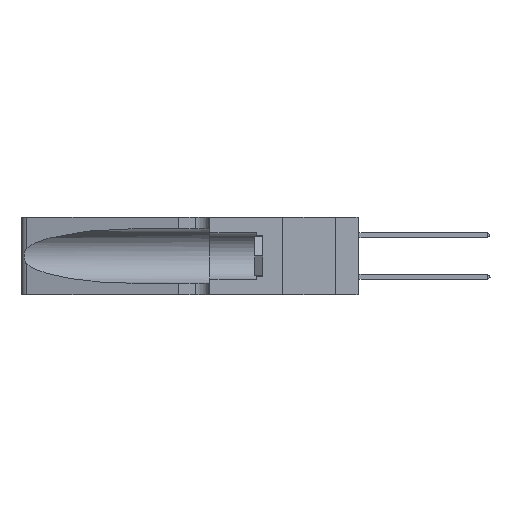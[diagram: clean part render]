
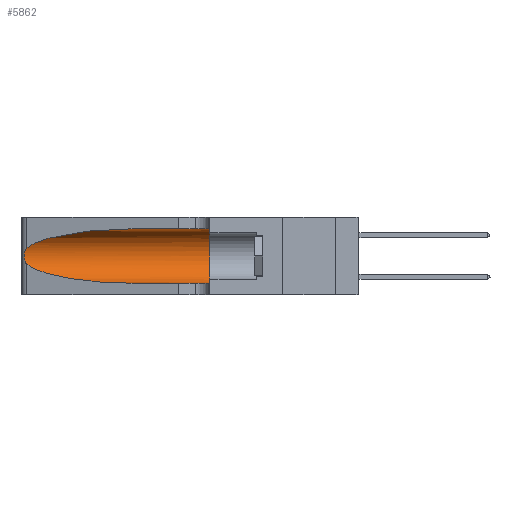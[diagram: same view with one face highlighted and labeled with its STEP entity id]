
A CAD part, left-side view. The second image highlights one B-rep face of the part: STEP entity #5862.
In plain terms, the highlighted cylindrical face has radius 3.308 mm (diameter 6.617 mm), a partial arc.
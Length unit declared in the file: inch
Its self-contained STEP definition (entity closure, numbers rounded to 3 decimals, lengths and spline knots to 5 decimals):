
#509 = CARTESIAN_POINT ( 'NONE',  ( 0.18966, 0.96281, 0.31525 ) ) ;
#884 = VECTOR ( 'NONE', #22544, 39.37008 ) ;
#1430 = ORIENTED_EDGE ( 'NONE', *, *, #12419, .T. ) ;
#1910 = LINE ( 'NONE', #32463, #884 ) ;
#2822 = AXIS2_PLACEMENT_3D ( 'NONE', #3629, #26888, #6989 ) ;
#3454 = CARTESIAN_POINT ( 'NONE',  ( 0.2373, 1.15595, 0.08982 ) ) ;
#3629 = CARTESIAN_POINT ( 'NONE',  ( 0.1305, 0.35, 0.185 ) ) ;
#3849 = CARTESIAN_POINT ( 'NONE',  ( 0.25487, 1.22718, 0.22369 ) ) ;
#4220 = CARTESIAN_POINT ( 'NONE',  ( 0.25787, 1.23484, 0.2124 ) ) ;
#4784 = ORIENTED_EDGE ( 'NONE', *, *, #43040, .T. ) ;
#4996 = EDGE_CURVE ( 'NONE', #33672, #31759, #29133, .T. ) ;
#5638 = B_SPLINE_CURVE_WITH_KNOTS ( 'NONE', 3,
 ( #17421, #37397, #24104, #4220, #27469, #7570, #30800, #10897, #34150, #14226, #37538, #17568, #40885, #20920 ),
 .UNSPECIFIED., .F., .F.,
 ( 4, 2, 2, 2, 2, 2, 4 ),
 ( 0., 0.00027, 0.00053, 0.00107, 0.0016, 0.00187, 0.00214 ),
 .UNSPECIFIED. ) ;
#5862 = ADVANCED_FACE ( 'NONE', ( #12404 ), #29058, .F. ) ;
#6635 = ORIENTED_EDGE ( 'NONE', *, *, #7661, .T. ) ;
#6989 = DIRECTION ( 'NONE',  ( 0., 0., 1. ) ) ;
#7570 = CARTESIAN_POINT ( 'NONE',  ( 0.26018, 1.23835, 0.19895 ) ) ;
#7661 = EDGE_CURVE ( 'NONE', #34881, #16072, #12007, .T. ) ;
#9265 = CARTESIAN_POINT ( 'NONE',  ( 0.1305, 1.61858, 0.31525 ) ) ;
#10110 = CARTESIAN_POINT ( 'NONE',  ( 0.25487, 1.22718, 0.14631 ) ) ;
#10220 = DIRECTION ( 'NONE',  ( 0., 0., -1. ) ) ;
#10897 = CARTESIAN_POINT ( 'NONE',  ( 0.26075, 1.23896, 0.178 ) ) ;
#11985 = EDGE_CURVE ( 'NONE', #33672, #36400, #32015, .T. ) ;
#12007 =( BOUNDED_CURVE ( )  B_SPLINE_CURVE ( 3, ( #10110, #3454, #30020, #13440 ),
 .UNSPECIFIED., .F., .F. ) 
 B_SPLINE_CURVE_WITH_KNOTS ( ( 4, 4 ),
 ( 3.44316, 4.71239 ),
 .UNSPECIFIED. ) 
 CURVE ( )  GEOMETRIC_REPRESENTATION_ITEM ( )  RATIONAL_B_SPLINE_CURVE ( ( 1., 0.87, 0.87, 1. ) ) 
 REPRESENTATION_ITEM ( '' )  );
#12404 = FACE_OUTER_BOUND ( 'NONE', #38258, .T. ) ;
#12419 = EDGE_CURVE ( 'NONE', #16072, #28475, #1910, .T. ) ;
#12459 = ORIENTED_EDGE ( 'NONE', *, *, #11985, .T. ) ;
#12831 = CARTESIAN_POINT ( 'NONE',  ( 0.1305, 0.35, 0.31525 ) ) ;
#13440 = CARTESIAN_POINT ( 'NONE',  ( 0.1305, 0.72297, 0.05475 ) ) ;
#14226 = CARTESIAN_POINT ( 'NONE',  ( 0.25856, 1.23593, 0.16098 ) ) ;
#14523 = CIRCLE ( 'NONE', #2822, 0.13025 ) ;
#16072 = VERTEX_POINT ( 'NONE', #16945 ) ;
#16945 = CARTESIAN_POINT ( 'NONE',  ( 0.1305, 0.72297, 0.05475 ) ) ;
#17421 = CARTESIAN_POINT ( 'NONE',  ( 0.25487, 1.22718, 0.22369 ) ) ;
#17568 = CARTESIAN_POINT ( 'NONE',  ( 0.25639, 1.23186, 0.15144 ) ) ;
#20098 = CARTESIAN_POINT ( 'NONE',  ( 0.1305, 1.61858, 0.185 ) ) ;
#20405 = CARTESIAN_POINT ( 'NONE',  ( 0.2373, 1.15595, 0.28018 ) ) ;
#20920 = CARTESIAN_POINT ( 'NONE',  ( 0.25487, 1.22718, 0.14631 ) ) ;
#22544 = DIRECTION ( 'NONE',  ( 0., -1., 0. ) ) ;
#24104 = CARTESIAN_POINT ( 'NONE',  ( 0.25639, 1.23184, 0.21858 ) ) ;
#26888 = DIRECTION ( 'NONE',  ( 0., 1., 0. ) ) ;
#27469 = CARTESIAN_POINT ( 'NONE',  ( 0.25854, 1.2359, 0.20912 ) ) ;
#28377 = CARTESIAN_POINT ( 'NONE',  ( 0.1305, 0.35, 0.05475 ) ) ;
#28475 = VERTEX_POINT ( 'NONE', #28377 ) ;
#29058 = CYLINDRICAL_SURFACE ( 'NONE', #32369, 0.13025 ) ;
#29133 = LINE ( 'NONE', #9265, #36973 ) ;
#30020 = CARTESIAN_POINT ( 'NONE',  ( 0.18966, 0.96281, 0.05475 ) ) ;
#30125 = DIRECTION ( 'NONE',  ( 0., -1., 0. ) ) ;
#30777 = ORIENTED_EDGE ( 'NONE', *, *, #4996, .F. ) ;
#30800 = CARTESIAN_POINT ( 'NONE',  ( 0.26075, 1.23896, 0.19203 ) ) ;
#31759 = VERTEX_POINT ( 'NONE', #12831 ) ;
#32015 =( BOUNDED_CURVE ( )  B_SPLINE_CURVE ( 3, ( #40357, #509, #20405, #3849 ),
 .UNSPECIFIED., .F., .F. ) 
 B_SPLINE_CURVE_WITH_KNOTS ( ( 4, 4 ),
 ( 1.5708, 2.84003 ),
 .UNSPECIFIED. ) 
 CURVE ( )  GEOMETRIC_REPRESENTATION_ITEM ( )  RATIONAL_B_SPLINE_CURVE ( ( 1., 0.87, 0.87, 1. ) ) 
 REPRESENTATION_ITEM ( '' )  );
#32369 = AXIS2_PLACEMENT_3D ( 'NONE', #20098, #30125, #10220 ) ;
#32463 = CARTESIAN_POINT ( 'NONE',  ( 0.1305, 1.61858, 0.05475 ) ) ;
#32638 = EDGE_CURVE ( 'NONE', #31759, #28475, #14523, .T. ) ;
#33672 = VERTEX_POINT ( 'NONE', #38605 ) ;
#34043 = ORIENTED_EDGE ( 'NONE', *, *, #32638, .F. ) ;
#34150 = CARTESIAN_POINT ( 'NONE',  ( 0.26017, 1.23833, 0.17102 ) ) ;
#34881 = VERTEX_POINT ( 'NONE', #37123 ) ;
#36400 = VERTEX_POINT ( 'NONE', #41222 ) ;
#36973 = VECTOR ( 'NONE', #39239, 39.37008 ) ;
#37123 = CARTESIAN_POINT ( 'NONE',  ( 0.25487, 1.22718, 0.14631 ) ) ;
#37397 = CARTESIAN_POINT ( 'NONE',  ( 0.25555, 1.22994, 0.2215 ) ) ;
#37538 = CARTESIAN_POINT ( 'NONE',  ( 0.25789, 1.23486, 0.15765 ) ) ;
#38258 = EDGE_LOOP ( 'NONE', ( #12459, #4784, #6635, #1430, #34043, #30777 ) ) ;
#38605 = CARTESIAN_POINT ( 'NONE',  ( 0.1305, 0.72297, 0.31525 ) ) ;
#39239 = DIRECTION ( 'NONE',  ( 0., -1., 0. ) ) ;
#40357 = CARTESIAN_POINT ( 'NONE',  ( 0.1305, 0.72297, 0.31525 ) ) ;
#40885 = CARTESIAN_POINT ( 'NONE',  ( 0.25555, 1.22993, 0.14849 ) ) ;
#41222 = CARTESIAN_POINT ( 'NONE',  ( 0.25487, 1.22718, 0.22369 ) ) ;
#43040 = EDGE_CURVE ( 'NONE', #36400, #34881, #5638, .T. ) ;
